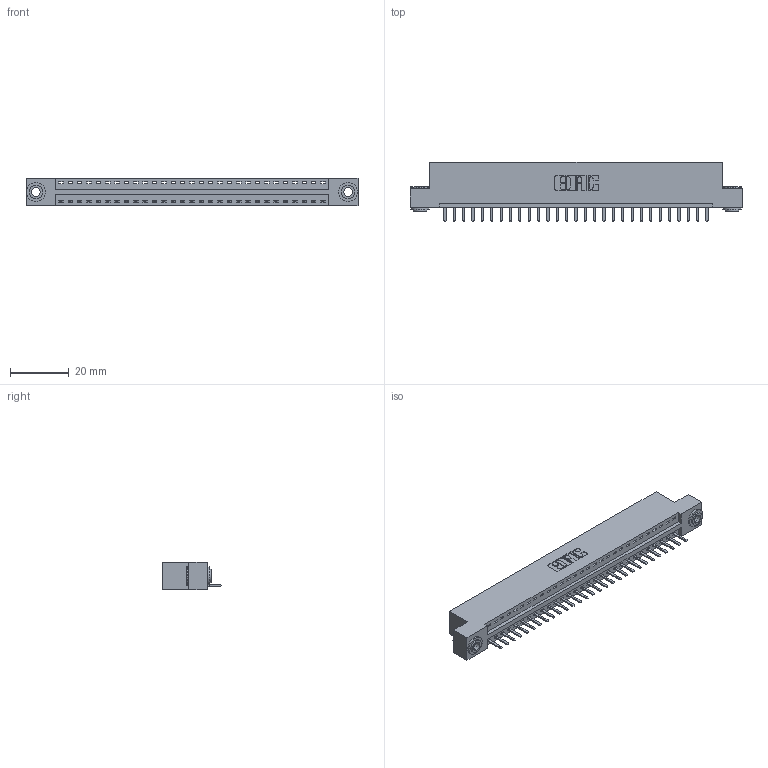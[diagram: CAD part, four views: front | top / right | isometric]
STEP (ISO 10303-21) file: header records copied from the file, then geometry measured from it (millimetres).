
FILE_DESCRIPTION (( 'STEP AP203' ), '1' );
FILE_NAME ('346-029-520-103.STEP', '2022-05-06T08:22:05', ( '' ), ( '' ), 'SwSTEP 2.0', 'SolidWorks 2020', '' );
FILE_SCHEMA (( 'CONFIG_CONTROL_DESIGN' ));
Length unit declared in the file: inch
Products named in the file (4): 345-292-001_345-293-120; 345-250-002_345-250-002-102; 346-029-520-103; 346 Part_Flush Mounting Lugs - 0.156 Dia-TH
Assembly tree (32 placements, depth 2):
  346-029-520-103
    346 Part_Flush Mounting Lugs - 0.156 Dia-TH
    345-292-001_345-293-120  x29
    345-250-002_345-250-002-102  x2
Bounding box: 112.65 x 20.02 x 9.4 mm (x, y, z)
Volume: 10611.3 mm3; surface area: 13095.5 mm2
Topology: 32 solids, 32 shells, 1972 faces, 5777 edges, 3770 vertices
Faces by surface type: plane 1318, cylinder 646, cone 8
Entity records: 20928 total; most frequent: CARTESIAN_POINT 3584, ORIENTED_EDGE 3526, DIRECTION 3195, EDGE_CURVE 1763, LINE 1487, VECTOR 1487, VERTEX_POINT 1170, AXIS2_PLACEMENT_3D 854
